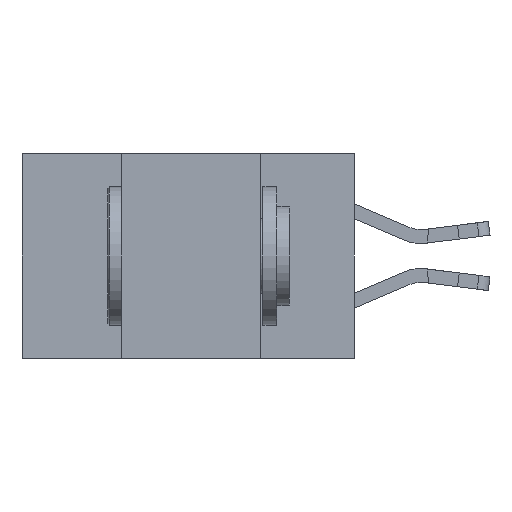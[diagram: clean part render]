
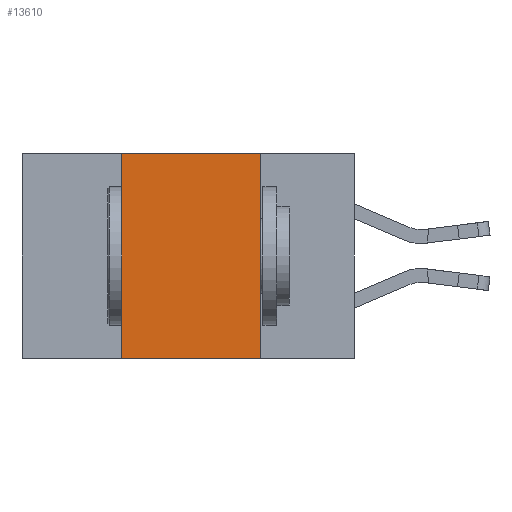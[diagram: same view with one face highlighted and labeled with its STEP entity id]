
A CAD part, left-side view. The second image highlights one B-rep face of the part: STEP entity #13610.
In plain terms, the highlighted planar face has unit normal (-1, 0, 0).
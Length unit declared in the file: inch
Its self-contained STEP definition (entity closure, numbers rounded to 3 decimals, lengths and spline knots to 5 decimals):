
#1724 = ORIENTED_EDGE ( 'NONE', *, *, #11309, .F. ) ;
#1738 = EDGE_CURVE ( 'NONE', #2205, #12559, #4952, .T. ) ;
#2205 = VERTEX_POINT ( 'NONE', #9569 ) ;
#2230 = LINE ( 'NONE', #4640, #12113 ) ;
#2341 = VECTOR ( 'NONE', #13824, 39.37008 ) ;
#3264 = VECTOR ( 'NONE', #6957, 39.37008 ) ;
#3618 = CARTESIAN_POINT ( 'NONE',  ( 0., 0.17, -0.37 ) ) ;
#3936 = EDGE_CURVE ( 'NONE', #5603, #2205, #6698, .T. ) ;
#4175 = LINE ( 'NONE', #8197, #2341 ) ;
#4238 = CARTESIAN_POINT ( 'NONE',  ( 0., 0.42, 0. ) ) ;
#4640 = CARTESIAN_POINT ( 'NONE',  ( 0., 0.6, -0.37 ) ) ;
#4952 = LINE ( 'NONE', #13036, #9275 ) ;
#5015 = ORIENTED_EDGE ( 'NONE', *, *, #14156, .T. ) ;
#5036 = EDGE_LOOP ( 'NONE', ( #5600, #10626, #1724, #5015 ) ) ;
#5134 = DIRECTION ( 'NONE',  ( 1., 0., 0. ) ) ;
#5465 = VERTEX_POINT ( 'NONE', #10230 ) ;
#5600 = ORIENTED_EDGE ( 'NONE', *, *, #1738, .F. ) ;
#5603 = VERTEX_POINT ( 'NONE', #4238 ) ;
#6611 = DIRECTION ( 'NONE',  ( 0., 0., -1. ) ) ;
#6698 = LINE ( 'NONE', #12125, #3264 ) ;
#6957 = DIRECTION ( 'NONE',  ( 0., -1., 0. ) ) ;
#7535 = DIRECTION ( 'NONE',  ( 0., -1., 0. ) ) ;
#8197 = CARTESIAN_POINT ( 'NONE',  ( 0., 0.42, -0.37 ) ) ;
#9275 = VECTOR ( 'NONE', #6611, 39.37008 ) ;
#9569 = CARTESIAN_POINT ( 'NONE',  ( 0., 0.17, 0. ) ) ;
#10230 = CARTESIAN_POINT ( 'NONE',  ( 0., 0.42, -0.37 ) ) ;
#10626 = ORIENTED_EDGE ( 'NONE', *, *, #3936, .F. ) ;
#11309 = EDGE_CURVE ( 'NONE', #5465, #5603, #4175, .T. ) ;
#12113 = VECTOR ( 'NONE', #7535, 39.37008 ) ;
#12125 = CARTESIAN_POINT ( 'NONE',  ( 0., 0.6, 0. ) ) ;
#12559 = VERTEX_POINT ( 'NONE', #3618 ) ;
#13036 = CARTESIAN_POINT ( 'NONE',  ( 0., 0.17, -0.37 ) ) ;
#13128 = FACE_OUTER_BOUND ( 'NONE', #5036, .T. ) ;
#13610 = ADVANCED_FACE ( 'NONE', ( #13128 ), #15996, .F. ) ;
#13824 = DIRECTION ( 'NONE',  ( 0., 0., 1. ) ) ;
#14156 = EDGE_CURVE ( 'NONE', #5465, #12559, #2230, .T. ) ;
#14197 = CARTESIAN_POINT ( 'NONE',  ( 0., 0.6, 0. ) ) ;
#15905 = DIRECTION ( 'NONE',  ( 0., 0., -1. ) ) ;
#15996 = PLANE ( 'NONE',  #16663 ) ;
#16663 = AXIS2_PLACEMENT_3D ( 'NONE', #14197, #5134, #15905 ) ;
